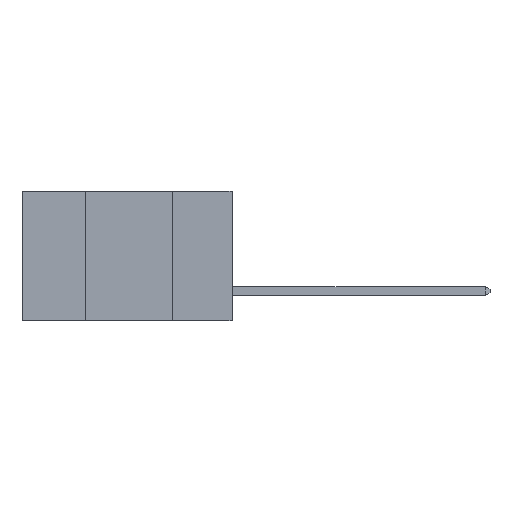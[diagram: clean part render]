
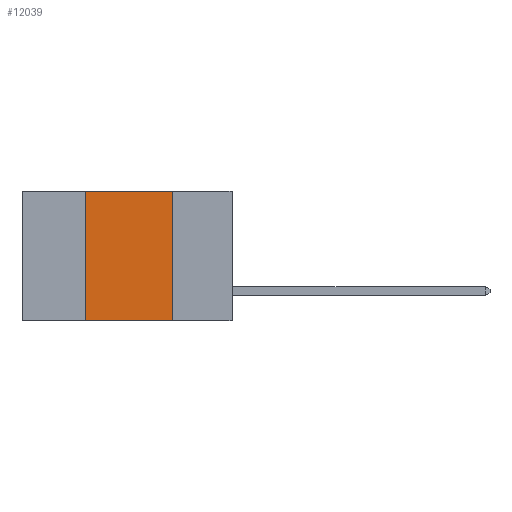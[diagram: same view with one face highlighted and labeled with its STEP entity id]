
A CAD part, left-side view. The second image highlights one B-rep face of the part: STEP entity #12039.
In plain terms, the highlighted planar face has unit normal (-1, 0, 0).
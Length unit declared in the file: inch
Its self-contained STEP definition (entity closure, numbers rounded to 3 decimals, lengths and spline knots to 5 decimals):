
#154 = CARTESIAN_POINT ( 'NONE',  ( 0., 0.42, 0. ) ) ;
#157 = EDGE_CURVE ( 'NONE', #1741, #983, #9021, .T. ) ;
#227 = DIRECTION ( 'NONE',  ( 0., -1., 0. ) ) ;
#824 = CARTESIAN_POINT ( 'NONE',  ( 0., 0.42, 0. ) ) ;
#983 = VERTEX_POINT ( 'NONE', #4390 ) ;
#1741 = VERTEX_POINT ( 'NONE', #2212 ) ;
#2212 = CARTESIAN_POINT ( 'NONE',  ( 0., 0.17, 0. ) ) ;
#2363 = VERTEX_POINT ( 'NONE', #11331 ) ;
#3979 = VECTOR ( 'NONE', #227, 39.37008 ) ;
#4280 = ORIENTED_EDGE ( 'NONE', *, *, #8880, .F. ) ;
#4361 = CARTESIAN_POINT ( 'NONE',  ( 0., 0.6, 0. ) ) ;
#4390 = CARTESIAN_POINT ( 'NONE',  ( 0., 0.17, -0.37 ) ) ;
#4436 = EDGE_LOOP ( 'NONE', ( #9095, #7325, #4280, #6701 ) ) ;
#4677 = LINE ( 'NONE', #11346, #9680 ) ;
#5590 = DIRECTION ( 'NONE',  ( 0., 0., -1. ) ) ;
#5640 = CARTESIAN_POINT ( 'NONE',  ( 0., 0.17, 0. ) ) ;
#6383 = VECTOR ( 'NONE', #9805, 39.37008 ) ;
#6396 = DIRECTION ( 'NONE',  ( 0., 0., -1. ) ) ;
#6701 = ORIENTED_EDGE ( 'NONE', *, *, #11218, .T. ) ;
#6914 = LINE ( 'NONE', #11032, #3979 ) ;
#7325 = ORIENTED_EDGE ( 'NONE', *, *, #8224, .F. ) ;
#7459 = AXIS2_PLACEMENT_3D ( 'NONE', #4361, #11663, #6396 ) ;
#8224 = EDGE_CURVE ( 'NONE', #9645, #1741, #4677, .T. ) ;
#8478 = FACE_OUTER_BOUND ( 'NONE', #4436, .T. ) ;
#8734 = VECTOR ( 'NONE', #5590, 39.37008 ) ;
#8795 = DIRECTION ( 'NONE',  ( 0., -1., 0. ) ) ;
#8856 = LINE ( 'NONE', #824, #6383 ) ;
#8880 = EDGE_CURVE ( 'NONE', #2363, #9645, #8856, .T. ) ;
#9021 = LINE ( 'NONE', #5640, #8734 ) ;
#9095 = ORIENTED_EDGE ( 'NONE', *, *, #157, .F. ) ;
#9645 = VERTEX_POINT ( 'NONE', #154 ) ;
#9680 = VECTOR ( 'NONE', #8795, 39.37008 ) ;
#9805 = DIRECTION ( 'NONE',  ( 0., 0., 1. ) ) ;
#10878 = PLANE ( 'NONE',  #7459 ) ;
#11032 = CARTESIAN_POINT ( 'NONE',  ( 0., 0.6, -0.37 ) ) ;
#11218 = EDGE_CURVE ( 'NONE', #2363, #983, #6914, .T. ) ;
#11331 = CARTESIAN_POINT ( 'NONE',  ( 0., 0.42, -0.37 ) ) ;
#11346 = CARTESIAN_POINT ( 'NONE',  ( 0., 0.6, 0. ) ) ;
#11663 = DIRECTION ( 'NONE',  ( 1., 0., 0. ) ) ;
#12039 = ADVANCED_FACE ( 'NONE', ( #8478 ), #10878, .F. ) ;
